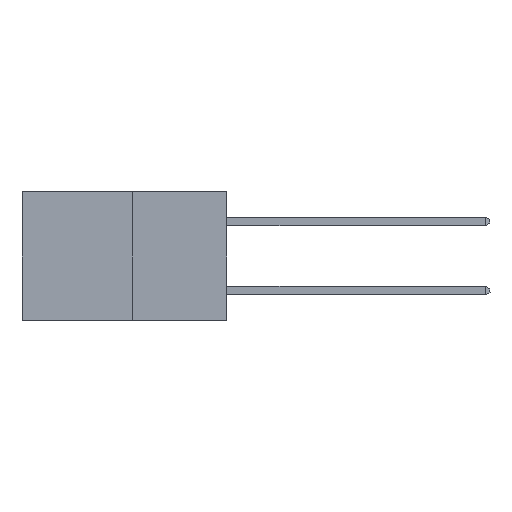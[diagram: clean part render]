
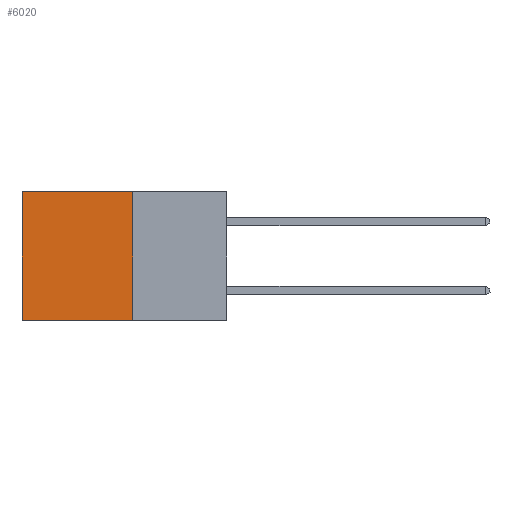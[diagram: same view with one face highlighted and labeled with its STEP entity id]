
A CAD part, left-side view. The second image highlights one B-rep face of the part: STEP entity #6020.
In plain terms, the highlighted planar face has unit normal (-1, 0, 0).
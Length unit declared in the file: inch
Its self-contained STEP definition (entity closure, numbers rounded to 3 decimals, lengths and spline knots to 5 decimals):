
#145 = EDGE_CURVE ( 'NONE', #6250, #15718, #9504, .T. ) ;
#729 = CARTESIAN_POINT ( 'NONE',  ( 0.277, 0.59, 0. ) ) ;
#1904 = FACE_OUTER_BOUND ( 'NONE', #10663, .T. ) ;
#2741 = AXIS2_PLACEMENT_3D ( 'NONE', #9554, #10022, #9436 ) ;
#3504 = VECTOR ( 'NONE', #8978, 39.37008 ) ;
#4459 = ORIENTED_EDGE ( 'NONE', *, *, #30711, .T. ) ;
#5278 = ORIENTED_EDGE ( 'NONE', *, *, #28008, .F. ) ;
#5680 = CARTESIAN_POINT ( 'NONE',  ( 0.277, 0.27, -0.37 ) ) ;
#5865 = CARTESIAN_POINT ( 'NONE',  ( 0.277, 0.27, 0. ) ) ;
#6020 = ADVANCED_FACE ( 'NONE', ( #1904 ), #9479, .F. ) ;
#6250 = VERTEX_POINT ( 'NONE', #5865 ) ;
#6276 = ORIENTED_EDGE ( 'NONE', *, *, #30911, .T. ) ;
#8978 = DIRECTION ( 'NONE',  ( 0., 0., -1. ) ) ;
#9436 = DIRECTION ( 'NONE',  ( 0., 0., -1. ) ) ;
#9479 = PLANE ( 'NONE',  #2741 ) ;
#9504 = LINE ( 'NONE', #10944, #22955 ) ;
#9554 = CARTESIAN_POINT ( 'NONE',  ( 0.277, 0.27, -0.37 ) ) ;
#10022 = DIRECTION ( 'NONE',  ( 1., 0., 0. ) ) ;
#10663 = EDGE_LOOP ( 'NONE', ( #4459, #5278, #26890, #6276 ) ) ;
#10913 = DIRECTION ( 'NONE',  ( 0., 0., -1. ) ) ;
#10944 = CARTESIAN_POINT ( 'NONE',  ( 0.277, 0.27, -0.37 ) ) ;
#11247 = LINE ( 'NONE', #31343, #17542 ) ;
#11408 = VECTOR ( 'NONE', #14003, 39.37008 ) ;
#11672 = LINE ( 'NONE', #22383, #3504 ) ;
#13267 = CARTESIAN_POINT ( 'NONE',  ( 0.277, 0.27, -0.37 ) ) ;
#14003 = DIRECTION ( 'NONE',  ( 0., 1., 0. ) ) ;
#15132 = CARTESIAN_POINT ( 'NONE',  ( 0.277, 0.59, -0.37 ) ) ;
#15718 = VERTEX_POINT ( 'NONE', #13267 ) ;
#17542 = VECTOR ( 'NONE', #17913, 39.37008 ) ;
#17913 = DIRECTION ( 'NONE',  ( 0., 1., 0. ) ) ;
#22383 = CARTESIAN_POINT ( 'NONE',  ( 0.277, 0.59, -0.37 ) ) ;
#22955 = VECTOR ( 'NONE', #10913, 39.37008 ) ;
#26890 = ORIENTED_EDGE ( 'NONE', *, *, #145, .F. ) ;
#27418 = LINE ( 'NONE', #5680, #11408 ) ;
#28008 = EDGE_CURVE ( 'NONE', #15718, #30217, #27418, .T. ) ;
#30217 = VERTEX_POINT ( 'NONE', #15132 ) ;
#30711 = EDGE_CURVE ( 'NONE', #31352, #30217, #11672, .T. ) ;
#30911 = EDGE_CURVE ( 'NONE', #6250, #31352, #11247, .T. ) ;
#31343 = CARTESIAN_POINT ( 'NONE',  ( 0.277, 0.27, 0. ) ) ;
#31352 = VERTEX_POINT ( 'NONE', #729 ) ;
